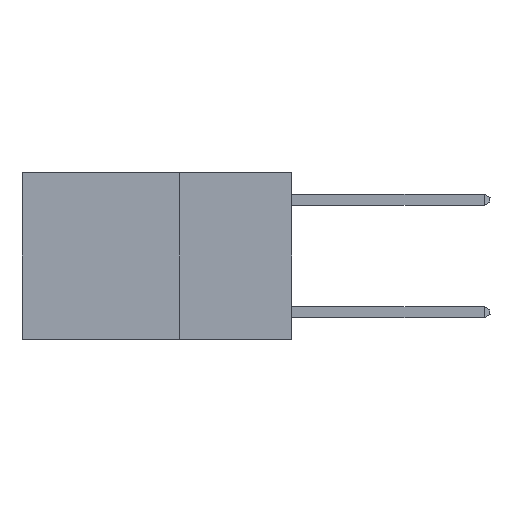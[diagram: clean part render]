
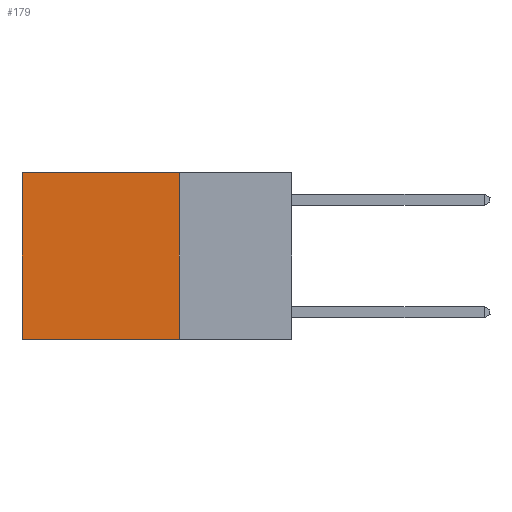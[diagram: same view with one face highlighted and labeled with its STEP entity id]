
A CAD part, left-side view. The second image highlights one B-rep face of the part: STEP entity #179.
In plain terms, the highlighted planar face has unit normal (-1, 0, 0).
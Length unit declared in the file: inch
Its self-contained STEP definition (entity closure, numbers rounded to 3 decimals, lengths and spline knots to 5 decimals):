
#179 = ADVANCED_FACE ( 'NONE', ( #1583 ), #12296, .F. ) ;
#253 = CARTESIAN_POINT ( 'NONE',  ( 0.2625, 0.25, 0. ) ) ;
#340 = VERTEX_POINT ( 'NONE', #9362 ) ;
#507 = VECTOR ( 'NONE', #10953, 39.37008 ) ;
#1301 = EDGE_LOOP ( 'NONE', ( #1405, #4454, #10883, #3568 ) ) ;
#1405 = ORIENTED_EDGE ( 'NONE', *, *, #1427, .T. ) ;
#1427 = EDGE_CURVE ( 'NONE', #340, #9806, #3204, .T. ) ;
#1449 = VECTOR ( 'NONE', #10853, 39.37008 ) ;
#1583 = FACE_OUTER_BOUND ( 'NONE', #1301, .T. ) ;
#1659 = CARTESIAN_POINT ( 'NONE',  ( 0.2625, 0.25, 0. ) ) ;
#1812 = LINE ( 'NONE', #10663, #10951 ) ;
#1984 = VERTEX_POINT ( 'NONE', #6477 ) ;
#3151 = LINE ( 'NONE', #3215, #7333 ) ;
#3204 = LINE ( 'NONE', #10015, #507 ) ;
#3215 = CARTESIAN_POINT ( 'NONE',  ( 0.2625, 0.25, 0. ) ) ;
#3568 = ORIENTED_EDGE ( 'NONE', *, *, #10474, .T. ) ;
#3926 = VERTEX_POINT ( 'NONE', #12469 ) ;
#4454 = ORIENTED_EDGE ( 'NONE', *, *, #9270, .F. ) ;
#4813 = AXIS2_PLACEMENT_3D ( 'NONE', #1659, #7474, #11340 ) ;
#6082 = LINE ( 'NONE', #253, #1449 ) ;
#6477 = CARTESIAN_POINT ( 'NONE',  ( 0.2625, 0.25, 0. ) ) ;
#7083 = DIRECTION ( 'NONE',  ( 0., 1., 0. ) ) ;
#7333 = VECTOR ( 'NONE', #7083, 39.37008 ) ;
#7474 = DIRECTION ( 'NONE',  ( 1., 0., 0. ) ) ;
#9270 = EDGE_CURVE ( 'NONE', #3926, #9806, #1812, .T. ) ;
#9362 = CARTESIAN_POINT ( 'NONE',  ( 0.2625, 0.6, 0. ) ) ;
#9730 = CARTESIAN_POINT ( 'NONE',  ( 0.2625, 0.6, -0.37 ) ) ;
#9806 = VERTEX_POINT ( 'NONE', #9730 ) ;
#10015 = CARTESIAN_POINT ( 'NONE',  ( 0.2625, 0.6, 0. ) ) ;
#10474 = EDGE_CURVE ( 'NONE', #1984, #340, #3151, .T. ) ;
#10663 = CARTESIAN_POINT ( 'NONE',  ( 0.2625, 0.25, -0.37 ) ) ;
#10853 = DIRECTION ( 'NONE',  ( 0., 0., -1. ) ) ;
#10883 = ORIENTED_EDGE ( 'NONE', *, *, #12049, .F. ) ;
#10951 = VECTOR ( 'NONE', #12424, 39.37008 ) ;
#10953 = DIRECTION ( 'NONE',  ( 0., 0., -1. ) ) ;
#11340 = DIRECTION ( 'NONE',  ( 0., 0., -1. ) ) ;
#12049 = EDGE_CURVE ( 'NONE', #1984, #3926, #6082, .T. ) ;
#12296 = PLANE ( 'NONE',  #4813 ) ;
#12424 = DIRECTION ( 'NONE',  ( 0., 1., 0. ) ) ;
#12469 = CARTESIAN_POINT ( 'NONE',  ( 0.2625, 0.25, -0.37 ) ) ;
